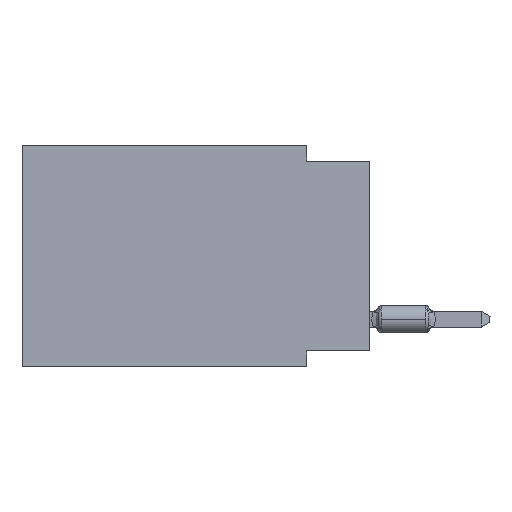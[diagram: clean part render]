
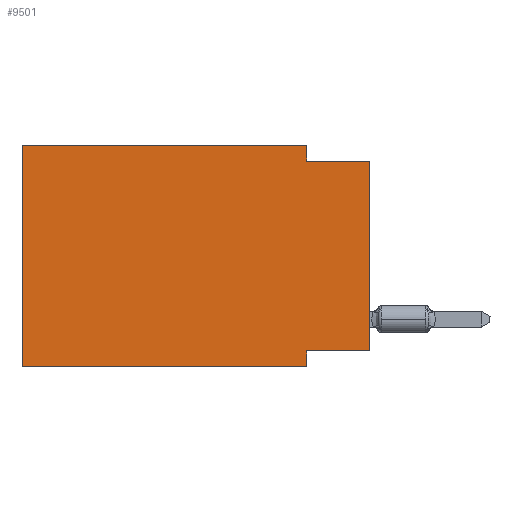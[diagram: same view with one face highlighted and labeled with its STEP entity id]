
A CAD part, left-side view. The second image highlights one B-rep face of the part: STEP entity #9501.
In plain terms, the highlighted planar face has unit normal (-1, 0, 0).
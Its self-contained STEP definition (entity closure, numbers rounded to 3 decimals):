
#232 = AXIS2_PLACEMENT_3D ( 'NONE', #7781, #20593, #11533 ) ;
#418 = CARTESIAN_POINT ( 'NONE',  ( 0., 13.97, -8.89 ) ) ;
#1437 = VERTEX_POINT ( 'NONE', #38873 ) ;
#1699 = VECTOR ( 'NONE', #42330, 1000. ) ;
#1820 = VECTOR ( 'NONE', #21821, 1000. ) ;
#2715 = CARTESIAN_POINT ( 'NONE',  ( 0., 13.97, 0. ) ) ;
#3083 = DIRECTION ( 'NONE',  ( 0., -1., 0. ) ) ;
#4654 = CARTESIAN_POINT ( 'NONE',  ( 0., 13.97, 0. ) ) ;
#6897 = EDGE_CURVE ( 'NONE', #36369, #1437, #38193, .T. ) ;
#7344 = FACE_OUTER_BOUND ( 'NONE', #9597, .T. ) ;
#7781 = CARTESIAN_POINT ( 'NONE',  ( 0., 13.97, 0. ) ) ;
#8479 = VECTOR ( 'NONE', #14405, 1000. ) ;
#9501 = ADVANCED_FACE ( 'NONE', ( #7344 ), #37985, .F. ) ;
#9597 = EDGE_LOOP ( 'NONE', ( #21102, #33776, #13562, #34918, #23591, #18700, #38209, #24416 ) ) ;
#9624 = LINE ( 'NONE', #16025, #25912 ) ;
#10158 = CARTESIAN_POINT ( 'NONE',  ( 0., 13.97, -8.89 ) ) ;
#11533 = DIRECTION ( 'NONE',  ( 0., 0., -1. ) ) ;
#12667 = EDGE_CURVE ( 'NONE', #17459, #31070, #41237, .T. ) ;
#12951 = EDGE_CURVE ( 'NONE', #23206, #19903, #17399, .T. ) ;
#13562 = ORIENTED_EDGE ( 'NONE', *, *, #27599, .F. ) ;
#14405 = DIRECTION ( 'NONE',  ( 0., -1., 0. ) ) ;
#16025 = CARTESIAN_POINT ( 'NONE',  ( 0., 0., 0. ) ) ;
#16337 = LINE ( 'NONE', #29780, #29170 ) ;
#17399 = LINE ( 'NONE', #418, #37341 ) ;
#17459 = VERTEX_POINT ( 'NONE', #2715 ) ;
#18181 = DIRECTION ( 'NONE',  ( 0., 0., 1. ) ) ;
#18338 = CARTESIAN_POINT ( 'NONE',  ( 0., 2.54, 0. ) ) ;
#18700 = ORIENTED_EDGE ( 'NONE', *, *, #12951, .T. ) ;
#18937 = CARTESIAN_POINT ( 'NONE',  ( 0., 0., -8.255 ) ) ;
#19903 = VERTEX_POINT ( 'NONE', #32935 ) ;
#20405 = VECTOR ( 'NONE', #18181, 1000. ) ;
#20593 = DIRECTION ( 'NONE',  ( 1., 0., 0. ) ) ;
#20617 = LINE ( 'NONE', #27874, #20405 ) ;
#21102 = ORIENTED_EDGE ( 'NONE', *, *, #39775, .T. ) ;
#21821 = DIRECTION ( 'NONE',  ( 0., 1., 0. ) ) ;
#22516 = EDGE_CURVE ( 'NONE', #23206, #17459, #20617, .T. ) ;
#22589 = CARTESIAN_POINT ( 'NONE',  ( 0., 2.54, -8.255 ) ) ;
#23163 = DIRECTION ( 'NONE',  ( 0., 0., -1. ) ) ;
#23206 = VERTEX_POINT ( 'NONE', #10158 ) ;
#23591 = ORIENTED_EDGE ( 'NONE', *, *, #22516, .F. ) ;
#24416 = ORIENTED_EDGE ( 'NONE', *, *, #24663, .F. ) ;
#24663 = EDGE_CURVE ( 'NONE', #34205, #25639, #28860, .T. ) ;
#24965 = CARTESIAN_POINT ( 'NONE',  ( 0., 0., -0.635 ) ) ;
#25639 = VERTEX_POINT ( 'NONE', #22589 ) ;
#25912 = VECTOR ( 'NONE', #43540, 1000. ) ;
#26883 = VECTOR ( 'NONE', #31990, 1000. ) ;
#27599 = EDGE_CURVE ( 'NONE', #31070, #36369, #38822, .T. ) ;
#27801 = EDGE_CURVE ( 'NONE', #25639, #19903, #16337, .T. ) ;
#27874 = CARTESIAN_POINT ( 'NONE',  ( 0., 13.97, 0. ) ) ;
#28860 = LINE ( 'NONE', #18937, #1820 ) ;
#29170 = VECTOR ( 'NONE', #23163, 1000. ) ;
#29780 = CARTESIAN_POINT ( 'NONE',  ( 0., 2.54, -8.89 ) ) ;
#29910 = CARTESIAN_POINT ( 'NONE',  ( 0., 0., -8.255 ) ) ;
#31070 = VERTEX_POINT ( 'NONE', #31676 ) ;
#31676 = CARTESIAN_POINT ( 'NONE',  ( 0., 2.54, 0. ) ) ;
#31990 = DIRECTION ( 'NONE',  ( 0., -1., 0. ) ) ;
#32935 = CARTESIAN_POINT ( 'NONE',  ( 0., 2.54, -8.89 ) ) ;
#33776 = ORIENTED_EDGE ( 'NONE', *, *, #6897, .F. ) ;
#34205 = VERTEX_POINT ( 'NONE', #29910 ) ;
#34918 = ORIENTED_EDGE ( 'NONE', *, *, #12667, .F. ) ;
#35503 = CARTESIAN_POINT ( 'NONE',  ( 0., 2.54, -0.635 ) ) ;
#36369 = VERTEX_POINT ( 'NONE', #35503 ) ;
#37341 = VECTOR ( 'NONE', #3083, 1000. ) ;
#37985 = PLANE ( 'NONE',  #232 ) ;
#38193 = LINE ( 'NONE', #24965, #8479 ) ;
#38209 = ORIENTED_EDGE ( 'NONE', *, *, #27801, .F. ) ;
#38822 = LINE ( 'NONE', #18338, #1699 ) ;
#38873 = CARTESIAN_POINT ( 'NONE',  ( 0., 0., -0.635 ) ) ;
#39775 = EDGE_CURVE ( 'NONE', #34205, #1437, #9624, .T. ) ;
#41237 = LINE ( 'NONE', #4654, #26883 ) ;
#42330 = DIRECTION ( 'NONE',  ( 0., 0., -1. ) ) ;
#43540 = DIRECTION ( 'NONE',  ( 0., 0., 1. ) ) ;
